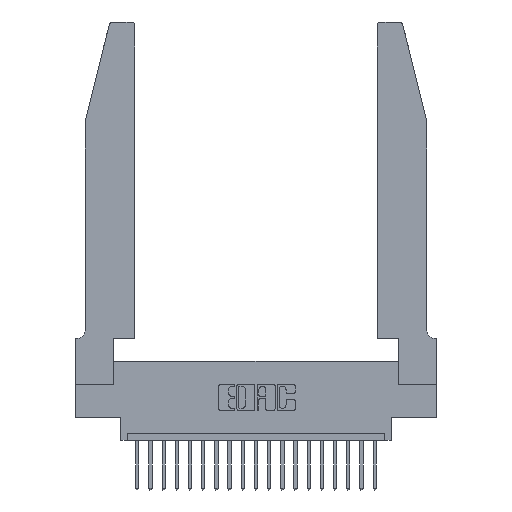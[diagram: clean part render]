
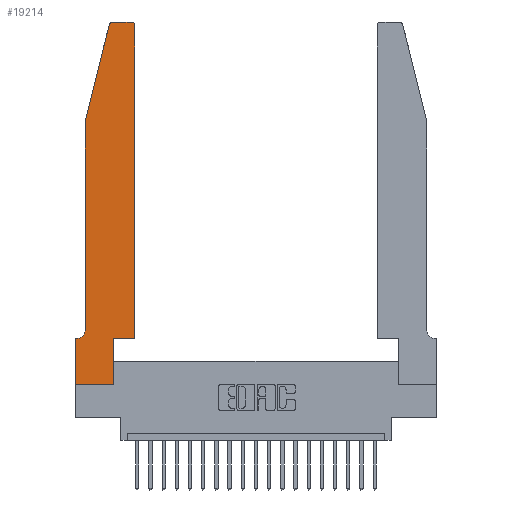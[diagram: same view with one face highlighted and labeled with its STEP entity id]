
A CAD part, top view. The second image highlights one B-rep face of the part: STEP entity #19214.
In plain terms, the highlighted planar face has unit normal (0, 0, 1).
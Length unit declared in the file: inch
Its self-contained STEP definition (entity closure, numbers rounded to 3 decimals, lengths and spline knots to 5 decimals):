
#135 = VECTOR ( 'NONE', #12318, 39.37008 ) ;
#308 = CARTESIAN_POINT ( 'NONE',  ( 0.4205, 2.75, 0.37 ) ) ;
#493 = LINE ( 'NONE', #14074, #16938 ) ;
#721 = EDGE_CURVE ( 'NONE', #21281, #6385, #19559, .T. ) ;
#2731 = ORIENTED_EDGE ( 'NONE', *, *, #18598, .T. ) ;
#2775 = DIRECTION ( 'NONE',  ( 0., 1., 0. ) ) ;
#2817 = VERTEX_POINT ( 'NONE', #14088 ) ;
#2902 = DIRECTION ( 'NONE',  ( 1., 0., 0. ) ) ;
#3195 = EDGE_CURVE ( 'NONE', #9260, #2817, #3566, .T. ) ;
#3221 = VECTOR ( 'NONE', #3922, 39.37008 ) ;
#3435 = VERTEX_POINT ( 'NONE', #17164 ) ;
#3531 = CARTESIAN_POINT ( 'NONE',  ( 0.4505, 0.35, 0.37 ) ) ;
#3566 = LINE ( 'NONE', #8219, #15693 ) ;
#3701 = PLANE ( 'NONE',  #9570 ) ;
#3716 = CARTESIAN_POINT ( 'NONE',  ( 0.2865, 0.35, 0.37 ) ) ;
#3753 = DIRECTION ( 'NONE',  ( 0., 0., 1. ) ) ;
#3790 = DIRECTION ( 'NONE',  ( 0., 1., 0. ) ) ;
#3922 = DIRECTION ( 'NONE',  ( 0., -1., 0. ) ) ;
#4738 = LINE ( 'NONE', #6307, #20598 ) ;
#5136 = VERTEX_POINT ( 'NONE', #20053 ) ;
#5427 = DIRECTION ( 'NONE',  ( -1., 0., 0. ) ) ;
#5639 = VERTEX_POINT ( 'NONE', #13909 ) ;
#5683 = LINE ( 'NONE', #5779, #11317 ) ;
#5779 = CARTESIAN_POINT ( 'NONE',  ( 0.4505, 0.35, 0.37 ) ) ;
#5816 = EDGE_CURVE ( 'NONE', #2817, #3435, #22318, .T. ) ;
#5931 = CARTESIAN_POINT ( 'NONE',  ( 0.0755, 2., 0.37 ) ) ;
#6307 = CARTESIAN_POINT ( 'NONE',  ( 0.0755, 2., 0.37 ) ) ;
#6385 = VERTEX_POINT ( 'NONE', #10547 ) ;
#7291 = DIRECTION ( 'NONE',  ( 0., 0., 1. ) ) ;
#7782 = EDGE_CURVE ( 'NONE', #9935, #11648, #21665, .T. ) ;
#8002 = CARTESIAN_POINT ( 'NONE',  ( 0.2865, 0.35, 0.37 ) ) ;
#8219 = CARTESIAN_POINT ( 'NONE',  ( 0.2605, 2.75, 0.37 ) ) ;
#8460 = ORIENTED_EDGE ( 'NONE', *, *, #3195, .T. ) ;
#8672 = ORIENTED_EDGE ( 'NONE', *, *, #721, .T. ) ;
#8916 = ORIENTED_EDGE ( 'NONE', *, *, #15413, .T. ) ;
#9075 = DIRECTION ( 'NONE',  ( -1., 0., 0. ) ) ;
#9260 = VERTEX_POINT ( 'NONE', #308 ) ;
#9570 = AXIS2_PLACEMENT_3D ( 'NONE', #17608, #7291, #19313 ) ;
#9713 = CARTESIAN_POINT ( 'NONE',  ( 0., 0., 0.37 ) ) ;
#9714 = CARTESIAN_POINT ( 'NONE',  ( 0., 0., 0.37 ) ) ;
#9822 = ORIENTED_EDGE ( 'NONE', *, *, #11661, .T. ) ;
#9893 = CARTESIAN_POINT ( 'NONE',  ( 0.4505, 2.72, 0.37 ) ) ;
#9924 = FACE_OUTER_BOUND ( 'NONE', #13352, .T. ) ;
#9935 = VERTEX_POINT ( 'NONE', #5931 ) ;
#10547 = CARTESIAN_POINT ( 'NONE',  ( 0.2865, 0., 0.37 ) ) ;
#11317 = VECTOR ( 'NONE', #2775, 39.37008 ) ;
#11572 = VECTOR ( 'NONE', #3790, 39.37008 ) ;
#11648 = VERTEX_POINT ( 'NONE', #14203 ) ;
#11661 = EDGE_CURVE ( 'NONE', #11648, #5136, #13108, .T. ) ;
#12318 = DIRECTION ( 'NONE',  ( 1., 0., 0. ) ) ;
#12396 = CARTESIAN_POINT ( 'NONE',  ( 0.4505, 0.35, 0.37 ) ) ;
#12471 = ORIENTED_EDGE ( 'NONE', *, *, #18492, .T. ) ;
#12914 = LINE ( 'NONE', #3716, #11572 ) ;
#12974 = DIRECTION ( 'NONE',  ( 0., -1., 0. ) ) ;
#13108 = CIRCLE ( 'NONE', #21887, 0.07 ) ;
#13206 = VERTEX_POINT ( 'NONE', #9893 ) ;
#13352 = EDGE_LOOP ( 'NONE', ( #8460, #14869, #15690, #17802, #9822, #19911, #14245, #8672, #2731, #16301, #8916, #12471 ) ) ;
#13567 = DIRECTION ( 'NONE',  ( 1., 0., 0. ) ) ;
#13909 = CARTESIAN_POINT ( 'NONE',  ( 0., 0.35, 0.37 ) ) ;
#14017 = VERTEX_POINT ( 'NONE', #8002 ) ;
#14054 = CARTESIAN_POINT ( 'NONE',  ( 0.284, 2.72, 0.37 ) ) ;
#14074 = CARTESIAN_POINT ( 'NONE',  ( 0.0755, 0.35, 0.37 ) ) ;
#14088 = CARTESIAN_POINT ( 'NONE',  ( 0.284, 2.75, 0.37 ) ) ;
#14140 = CARTESIAN_POINT ( 'NONE',  ( 0., 0., 0.37 ) ) ;
#14203 = CARTESIAN_POINT ( 'NONE',  ( 0.0755, 0.42, 0.37 ) ) ;
#14226 = LINE ( 'NONE', #14140, #3221 ) ;
#14245 = ORIENTED_EDGE ( 'NONE', *, *, #19175, .T. ) ;
#14412 = LINE ( 'NONE', #12396, #135 ) ;
#14869 = ORIENTED_EDGE ( 'NONE', *, *, #5816, .T. ) ;
#15413 = EDGE_CURVE ( 'NONE', #17967, #13206, #5683, .T. ) ;
#15690 = ORIENTED_EDGE ( 'NONE', *, *, #21774, .T. ) ;
#15693 = VECTOR ( 'NONE', #20096, 39.37008 ) ;
#15781 = DIRECTION ( 'NONE',  ( 1., 0., 0. ) ) ;
#15999 = VECTOR ( 'NONE', #12974, 39.37008 ) ;
#16301 = ORIENTED_EDGE ( 'NONE', *, *, #22034, .T. ) ;
#16694 = CIRCLE ( 'NONE', #18089, 0.03 ) ;
#16938 = VECTOR ( 'NONE', #5427, 39.37008 ) ;
#17164 = CARTESIAN_POINT ( 'NONE',  ( 0.25487, 2.72718, 0.37 ) ) ;
#17254 = DIRECTION ( 'NONE',  ( 0., 0., 1. ) ) ;
#17608 = CARTESIAN_POINT ( 'NONE',  ( 0., 0.35, 0.37 ) ) ;
#17802 = ORIENTED_EDGE ( 'NONE', *, *, #7782, .T. ) ;
#17967 = VERTEX_POINT ( 'NONE', #3531 ) ;
#18089 = AXIS2_PLACEMENT_3D ( 'NONE', #22295, #17254, #13567 ) ;
#18198 = DIRECTION ( 'NONE',  ( -0.239, -0.971, 0. ) ) ;
#18492 = EDGE_CURVE ( 'NONE', #13206, #9260, #16694, .T. ) ;
#18598 = EDGE_CURVE ( 'NONE', #6385, #14017, #12914, .T. ) ;
#19031 = VECTOR ( 'NONE', #2902, 39.37008 ) ;
#19175 = EDGE_CURVE ( 'NONE', #5639, #21281, #14226, .T. ) ;
#19179 = EDGE_CURVE ( 'NONE', #5136, #5639, #493, .T. ) ;
#19214 = ADVANCED_FACE ( 'NONE', ( #9924 ), #3701, .T. ) ;
#19313 = DIRECTION ( 'NONE',  ( 1., 0., 0. ) ) ;
#19385 = DIRECTION ( 'NONE',  ( 0., 0., -1. ) ) ;
#19458 = CARTESIAN_POINT ( 'NONE',  ( 0.0055, 0.42, 0.37 ) ) ;
#19559 = LINE ( 'NONE', #9714, #19031 ) ;
#19911 = ORIENTED_EDGE ( 'NONE', *, *, #19179, .T. ) ;
#20053 = CARTESIAN_POINT ( 'NONE',  ( 0.0055, 0.35, 0.37 ) ) ;
#20096 = DIRECTION ( 'NONE',  ( -1., 0., 0. ) ) ;
#20598 = VECTOR ( 'NONE', #18198, 39.37008 ) ;
#21281 = VERTEX_POINT ( 'NONE', #9713 ) ;
#21629 = CARTESIAN_POINT ( 'NONE',  ( 0.0755, 2., 0.37 ) ) ;
#21647 = AXIS2_PLACEMENT_3D ( 'NONE', #14054, #3753, #15781 ) ;
#21665 = LINE ( 'NONE', #21629, #15999 ) ;
#21774 = EDGE_CURVE ( 'NONE', #3435, #9935, #4738, .T. ) ;
#21887 = AXIS2_PLACEMENT_3D ( 'NONE', #19458, #19385, #9075 ) ;
#22034 = EDGE_CURVE ( 'NONE', #14017, #17967, #14412, .T. ) ;
#22295 = CARTESIAN_POINT ( 'NONE',  ( 0.4205, 2.72, 0.37 ) ) ;
#22318 = CIRCLE ( 'NONE', #21647, 0.03 ) ;
